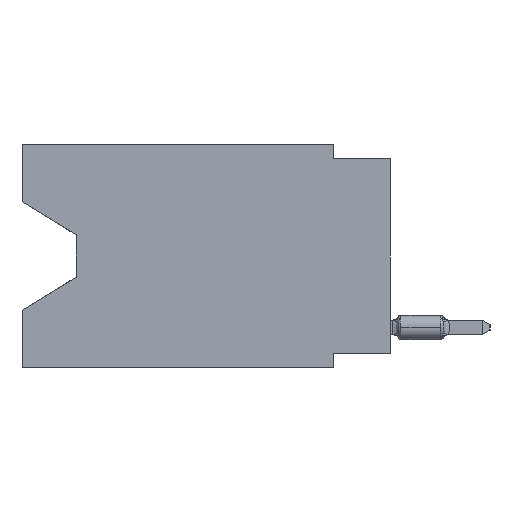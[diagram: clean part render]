
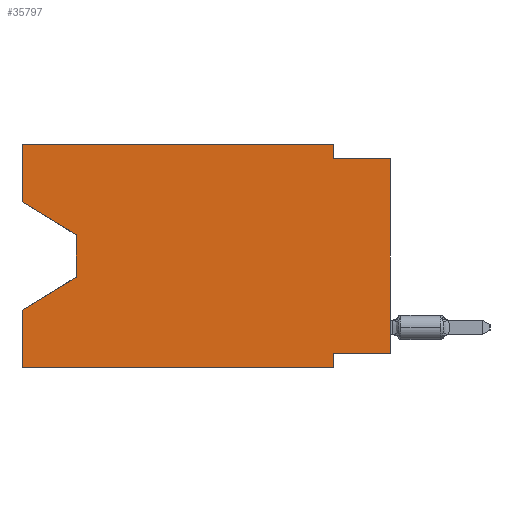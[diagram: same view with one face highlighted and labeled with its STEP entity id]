
A CAD part, left-side view. The second image highlights one B-rep face of the part: STEP entity #35797.
In plain terms, the highlighted planar face has unit normal (-1, 0, 0).
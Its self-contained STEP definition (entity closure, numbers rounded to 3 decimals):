
#992 = ORIENTED_EDGE ( 'NONE', *, *, #13312, .T. ) ;
#1623 = VERTEX_POINT ( 'NONE', #21728 ) ;
#1677 = AXIS2_PLACEMENT_3D ( 'NONE', #14808, #31446, #32163 ) ;
#2604 = ORIENTED_EDGE ( 'NONE', *, *, #23567, .F. ) ;
#4023 = LINE ( 'NONE', #48233, #63782 ) ;
#4103 = EDGE_CURVE ( 'NONE', #35648, #8631, #60289, .T. ) ;
#5158 = DIRECTION ( 'NONE',  ( 0., 0., 1. ) ) ;
#5496 = LINE ( 'NONE', #60238, #14303 ) ;
#5631 = ORIENTED_EDGE ( 'NONE', *, *, #43030, .F. ) ;
#8631 = VERTEX_POINT ( 'NONE', #45041 ) ;
#8921 = ORIENTED_EDGE ( 'NONE', *, *, #65064, .T. ) ;
#10260 = EDGE_CURVE ( 'NONE', #42034, #1623, #63165, .T. ) ;
#10653 = CARTESIAN_POINT ( 'NONE',  ( 0., 16.383, -2.546 ) ) ;
#11569 = CARTESIAN_POINT ( 'NONE',  ( 0., 16.383, 0. ) ) ;
#13312 = EDGE_CURVE ( 'NONE', #66426, #48270, #63830, .T. ) ;
#13571 = VERTEX_POINT ( 'NONE', #11569 ) ;
#14303 = VECTOR ( 'NONE', #5158, 1000. ) ;
#14808 = CARTESIAN_POINT ( 'NONE',  ( 0., 16.383, 0. ) ) ;
#14895 = VECTOR ( 'NONE', #52606, 1000. ) ;
#15214 = CARTESIAN_POINT ( 'NONE',  ( 0., 2.54, 0. ) ) ;
#16235 = DIRECTION ( 'NONE',  ( 0., 0., -1. ) ) ;
#16293 = VERTEX_POINT ( 'NONE', #34242 ) ;
#17261 = CARTESIAN_POINT ( 'NONE',  ( 0., 2.54, -9.906 ) ) ;
#18083 = LINE ( 'NONE', #46336, #62366 ) ;
#18095 = VECTOR ( 'NONE', #28746, 1000. ) ;
#18489 = DIRECTION ( 'NONE',  ( 0., 0., -1. ) ) ;
#18532 = VERTEX_POINT ( 'NONE', #17261 ) ;
#18626 = VECTOR ( 'NONE', #16235, 1000. ) ;
#18883 = DIRECTION ( 'NONE',  ( 0., 0.855, -0.519 ) ) ;
#19456 = VECTOR ( 'NONE', #18883, 1000. ) ;
#20551 = ORIENTED_EDGE ( 'NONE', *, *, #4103, .T. ) ;
#21728 = CARTESIAN_POINT ( 'NONE',  ( 0., 2.54, -0.635 ) ) ;
#22799 = VERTEX_POINT ( 'NONE', #34429 ) ;
#23360 = VECTOR ( 'NONE', #32737, 1000. ) ;
#23567 = EDGE_CURVE ( 'NONE', #13571, #42034, #50957, .T. ) ;
#24395 = ORIENTED_EDGE ( 'NONE', *, *, #45453, .F. ) ;
#24871 = EDGE_CURVE ( 'NONE', #61164, #48270, #41718, .T. ) ;
#26975 = VECTOR ( 'NONE', #67912, 1000. ) ;
#27478 = CARTESIAN_POINT ( 'NONE',  ( 0., 16.383, -9.906 ) ) ;
#28025 = LINE ( 'NONE', #56314, #18095 ) ;
#28320 = ORIENTED_EDGE ( 'NONE', *, *, #39123, .T. ) ;
#28746 = DIRECTION ( 'NONE',  ( 0., -1., 0. ) ) ;
#29297 = DIRECTION ( 'NONE',  ( 0., 1., 0. ) ) ;
#29810 = CARTESIAN_POINT ( 'NONE',  ( 0., 13.97, -5.893 ) ) ;
#31446 = DIRECTION ( 'NONE',  ( 1., 0., 0. ) ) ;
#32163 = DIRECTION ( 'NONE',  ( 0., 0., -1. ) ) ;
#32737 = DIRECTION ( 'NONE',  ( 0., -0.855, -0.519 ) ) ;
#33895 = DIRECTION ( 'NONE',  ( 0., -1., 0. ) ) ;
#34242 = CARTESIAN_POINT ( 'NONE',  ( 0., 0., -9.271 ) ) ;
#34429 = CARTESIAN_POINT ( 'NONE',  ( 0., 2.54, -9.271 ) ) ;
#34770 = LINE ( 'NONE', #46034, #60621 ) ;
#35648 = VERTEX_POINT ( 'NONE', #64119 ) ;
#35797 = ADVANCED_FACE ( 'NONE', ( #48146 ), #42336, .F. ) ;
#36769 = EDGE_CURVE ( 'NONE', #35648, #13571, #5496, .T. ) ;
#37671 = VECTOR ( 'NONE', #56279, 1000. ) ;
#38525 = EDGE_LOOP ( 'NONE', ( #20551, #44463, #992, #49907, #28320, #56412, #24395, #8921, #5631, #67133, #2604, #64439 ) ) ;
#39123 = EDGE_CURVE ( 'NONE', #61164, #18532, #57707, .T. ) ;
#39553 = EDGE_CURVE ( 'NONE', #22799, #18532, #34770, .T. ) ;
#39947 = CARTESIAN_POINT ( 'NONE',  ( 0., 2.54, 0. ) ) ;
#41364 = VECTOR ( 'NONE', #33895, 1000. ) ;
#41718 = LINE ( 'NONE', #52954, #14895 ) ;
#42034 = VERTEX_POINT ( 'NONE', #15214 ) ;
#42336 = PLANE ( 'NONE',  #1677 ) ;
#43030 = EDGE_CURVE ( 'NONE', #1623, #62049, #28025, .T. ) ;
#43762 = LINE ( 'NONE', #65917, #18626 ) ;
#44463 = ORIENTED_EDGE ( 'NONE', *, *, #64897, .T. ) ;
#45041 = CARTESIAN_POINT ( 'NONE',  ( 0., 13.97, -4.013 ) ) ;
#45453 = EDGE_CURVE ( 'NONE', #16293, #22799, #18083, .T. ) ;
#46034 = CARTESIAN_POINT ( 'NONE',  ( 0., 2.54, -9.906 ) ) ;
#46336 = CARTESIAN_POINT ( 'NONE',  ( 0., 0., -9.271 ) ) ;
#48146 = FACE_OUTER_BOUND ( 'NONE', #38525, .T. ) ;
#48233 = CARTESIAN_POINT ( 'NONE',  ( 0., 0., 0. ) ) ;
#48270 = VERTEX_POINT ( 'NONE', #60933 ) ;
#49907 = ORIENTED_EDGE ( 'NONE', *, *, #24871, .F. ) ;
#50588 = CARTESIAN_POINT ( 'NONE',  ( 0., 16.383, 0. ) ) ;
#50957 = LINE ( 'NONE', #50588, #41364 ) ;
#52606 = DIRECTION ( 'NONE',  ( 0., 0., 1. ) ) ;
#52954 = CARTESIAN_POINT ( 'NONE',  ( 0., 16.383, 0. ) ) ;
#56279 = DIRECTION ( 'NONE',  ( 0., 0., -1. ) ) ;
#56314 = CARTESIAN_POINT ( 'NONE',  ( 0., 0., -0.635 ) ) ;
#56412 = ORIENTED_EDGE ( 'NONE', *, *, #39553, .F. ) ;
#56993 = CARTESIAN_POINT ( 'NONE',  ( 0., 16.383, -9.906 ) ) ;
#57707 = LINE ( 'NONE', #56993, #26975 ) ;
#58404 = DIRECTION ( 'NONE',  ( 0., 0., 1. ) ) ;
#60238 = CARTESIAN_POINT ( 'NONE',  ( 0., 16.383, 0. ) ) ;
#60289 = LINE ( 'NONE', #10653, #23360 ) ;
#60621 = VECTOR ( 'NONE', #18489, 1000. ) ;
#60933 = CARTESIAN_POINT ( 'NONE',  ( 0., 16.383, -7.36 ) ) ;
#61164 = VERTEX_POINT ( 'NONE', #27478 ) ;
#62049 = VERTEX_POINT ( 'NONE', #64228 ) ;
#62366 = VECTOR ( 'NONE', #29297, 1000. ) ;
#63165 = LINE ( 'NONE', #39947, #37671 ) ;
#63470 = CARTESIAN_POINT ( 'NONE',  ( 0., 13.97, -5.893 ) ) ;
#63782 = VECTOR ( 'NONE', #58404, 1000. ) ;
#63830 = LINE ( 'NONE', #63470, #19456 ) ;
#64119 = CARTESIAN_POINT ( 'NONE',  ( 0., 16.383, -2.546 ) ) ;
#64228 = CARTESIAN_POINT ( 'NONE',  ( 0., 0., -0.635 ) ) ;
#64439 = ORIENTED_EDGE ( 'NONE', *, *, #36769, .F. ) ;
#64897 = EDGE_CURVE ( 'NONE', #8631, #66426, #43762, .T. ) ;
#65064 = EDGE_CURVE ( 'NONE', #16293, #62049, #4023, .T. ) ;
#65917 = CARTESIAN_POINT ( 'NONE',  ( 0., 13.97, -4.013 ) ) ;
#66426 = VERTEX_POINT ( 'NONE', #29810 ) ;
#67133 = ORIENTED_EDGE ( 'NONE', *, *, #10260, .F. ) ;
#67912 = DIRECTION ( 'NONE',  ( 0., -1., 0. ) ) ;
